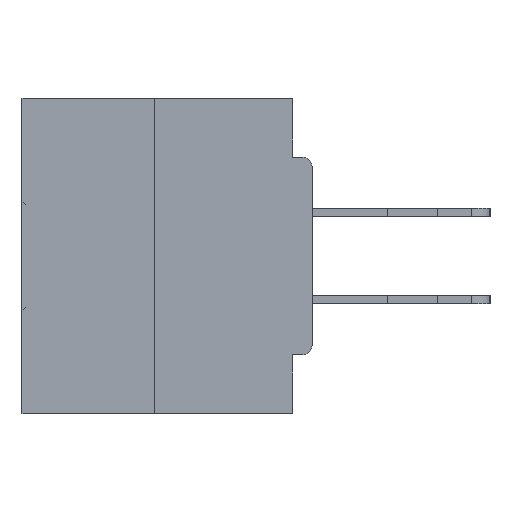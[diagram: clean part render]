
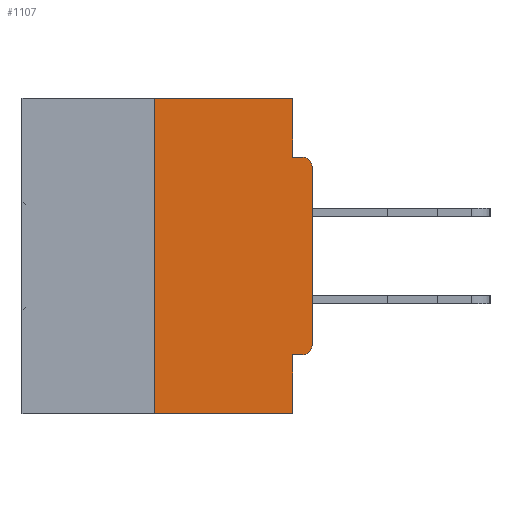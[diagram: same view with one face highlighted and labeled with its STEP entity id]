
A CAD part, left-side view. The second image highlights one B-rep face of the part: STEP entity #1107.
In plain terms, the highlighted planar face has unit normal (-1, 0, 0).
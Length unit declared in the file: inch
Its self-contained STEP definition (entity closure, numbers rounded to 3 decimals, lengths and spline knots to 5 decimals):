
#235 = VECTOR ( 'NONE', #36347, 39.37008 ) ;
#356 = VECTOR ( 'NONE', #8314, 39.37008 ) ;
#1107 = ADVANCED_FACE ( 'NONE', ( #28666 ), #30904, .F. ) ;
#2574 = CARTESIAN_POINT ( 'NONE',  ( 0., 0., -0.1085 ) ) ;
#3475 = DIRECTION ( 'NONE',  ( -1., 0., 0. ) ) ;
#3904 = VERTEX_POINT ( 'NONE', #31282 ) ;
#3958 = CARTESIAN_POINT ( 'NONE',  ( 0., 0.25, 0. ) ) ;
#4335 = DIRECTION ( 'NONE',  ( 1., 0., 0. ) ) ;
#4361 = ORIENTED_EDGE ( 'NONE', *, *, #42963, .T. ) ;
#5199 = AXIS2_PLACEMENT_3D ( 'NONE', #13605, #17382, #41067 ) ;
#5365 = VECTOR ( 'NONE', #28498, 39.37008 ) ;
#5649 = EDGE_CURVE ( 'NONE', #43180, #18150, #7087, .T. ) ;
#6334 = LINE ( 'NONE', #19129, #27477 ) ;
#7087 = LINE ( 'NONE', #37291, #10281 ) ;
#8314 = DIRECTION ( 'NONE',  ( 0., 1., 0. ) ) ;
#8985 = EDGE_CURVE ( 'NONE', #18150, #36351, #30164, .T. ) ;
#9647 = CARTESIAN_POINT ( 'NONE',  ( 0., 0.015, -0.4065 ) ) ;
#9792 = CARTESIAN_POINT ( 'NONE',  ( 0., 0.25, -0.5 ) ) ;
#9830 = EDGE_CURVE ( 'NONE', #14488, #33222, #6334, .T. ) ;
#10281 = VECTOR ( 'NONE', #16440, 39.37008 ) ;
#11903 = CIRCLE ( 'NONE', #30479, 0.015 ) ;
#11998 = LINE ( 'NONE', #24845, #24604 ) ;
#12230 = VERTEX_POINT ( 'NONE', #35843 ) ;
#13387 = EDGE_CURVE ( 'NONE', #33222, #12230, #39884, .T. ) ;
#13605 = CARTESIAN_POINT ( 'NONE',  ( 0., 0.015, -0.1085 ) ) ;
#13852 = DIRECTION ( 'NONE',  ( 0., 0., -1. ) ) ;
#14488 = VERTEX_POINT ( 'NONE', #9792 ) ;
#14993 = CARTESIAN_POINT ( 'NONE',  ( 0., 0.031, -0.5 ) ) ;
#14994 = EDGE_CURVE ( 'NONE', #16891, #36351, #37554, .T. ) ;
#15096 = CARTESIAN_POINT ( 'NONE',  ( 0., 0., -0.0935 ) ) ;
#16440 = DIRECTION ( 'NONE',  ( 0., 0., 1. ) ) ;
#16891 = VERTEX_POINT ( 'NONE', #23171 ) ;
#17126 = LINE ( 'NONE', #32949, #235 ) ;
#17382 = DIRECTION ( 'NONE',  ( -1., 0., 0. ) ) ;
#17494 = CARTESIAN_POINT ( 'NONE',  ( 0., 0.031, -0.5 ) ) ;
#18150 = VERTEX_POINT ( 'NONE', #2574 ) ;
#18290 = ORIENTED_EDGE ( 'NONE', *, *, #35519, .F. ) ;
#18487 = DIRECTION ( 'NONE',  ( 0., -1., 0. ) ) ;
#19129 = CARTESIAN_POINT ( 'NONE',  ( 0., 0.25, 0. ) ) ;
#20282 = ORIENTED_EDGE ( 'NONE', *, *, #8985, .T. ) ;
#23171 = CARTESIAN_POINT ( 'NONE',  ( 0., 0.031, -0.0935 ) ) ;
#24604 = VECTOR ( 'NONE', #39071, 39.37008 ) ;
#24845 = CARTESIAN_POINT ( 'NONE',  ( 0., 0.46, -0.5 ) ) ;
#25630 = EDGE_LOOP ( 'NONE', ( #43485, #36780, #4361, #28455, #18290, #30085, #40351, #20282, #36782, #35275 ) ) ;
#25725 = AXIS2_PLACEMENT_3D ( 'NONE', #31363, #4335, #37553 ) ;
#25814 = DIRECTION ( 'NONE',  ( 0., 0., 1. ) ) ;
#27001 = EDGE_CURVE ( 'NONE', #42233, #43180, #11903, .T. ) ;
#27413 = CARTESIAN_POINT ( 'NONE',  ( 0., 0.015, -0.3915 ) ) ;
#27477 = VECTOR ( 'NONE', #25814, 39.37008 ) ;
#28059 = VECTOR ( 'NONE', #31601, 39.37008 ) ;
#28455 = ORIENTED_EDGE ( 'NONE', *, *, #38924, .F. ) ;
#28498 = DIRECTION ( 'NONE',  ( 0., 0., -1. ) ) ;
#28666 = FACE_OUTER_BOUND ( 'NONE', #25630, .T. ) ;
#30085 = ORIENTED_EDGE ( 'NONE', *, *, #27001, .T. ) ;
#30164 = CIRCLE ( 'NONE', #5199, 0.015 ) ;
#30479 = AXIS2_PLACEMENT_3D ( 'NONE', #27413, #3475, #13852 ) ;
#30904 = PLANE ( 'NONE',  #25725 ) ;
#31282 = CARTESIAN_POINT ( 'NONE',  ( 0., 0.031, -0.4065 ) ) ;
#31363 = CARTESIAN_POINT ( 'NONE',  ( 0., 0.46, 0. ) ) ;
#31601 = DIRECTION ( 'NONE',  ( 0., -1., 0. ) ) ;
#32949 = CARTESIAN_POINT ( 'NONE',  ( 0., 0.031, 0. ) ) ;
#33222 = VERTEX_POINT ( 'NONE', #3958 ) ;
#33927 = CARTESIAN_POINT ( 'NONE',  ( 0., 0., -0.3915 ) ) ;
#35275 = ORIENTED_EDGE ( 'NONE', *, *, #36697, .F. ) ;
#35506 = LINE ( 'NONE', #17494, #5365 ) ;
#35519 = EDGE_CURVE ( 'NONE', #42233, #3904, #41652, .T. ) ;
#35843 = CARTESIAN_POINT ( 'NONE',  ( 0., 0.031, 0. ) ) ;
#36347 = DIRECTION ( 'NONE',  ( 0., 0., -1. ) ) ;
#36351 = VERTEX_POINT ( 'NONE', #39739 ) ;
#36697 = EDGE_CURVE ( 'NONE', #12230, #16891, #17126, .T. ) ;
#36780 = ORIENTED_EDGE ( 'NONE', *, *, #9830, .F. ) ;
#36782 = ORIENTED_EDGE ( 'NONE', *, *, #14994, .F. ) ;
#37291 = CARTESIAN_POINT ( 'NONE',  ( 0., 0., 0. ) ) ;
#37553 = DIRECTION ( 'NONE',  ( 0., 0., -1. ) ) ;
#37554 = LINE ( 'NONE', #15096, #28059 ) ;
#38172 = CARTESIAN_POINT ( 'NONE',  ( 0., 0., -0.4065 ) ) ;
#38635 = CARTESIAN_POINT ( 'NONE',  ( 0., 0.46, 0. ) ) ;
#38924 = EDGE_CURVE ( 'NONE', #3904, #42444, #35506, .T. ) ;
#39071 = DIRECTION ( 'NONE',  ( 0., -1., 0. ) ) ;
#39739 = CARTESIAN_POINT ( 'NONE',  ( 0., 0.015, -0.0935 ) ) ;
#39884 = LINE ( 'NONE', #38635, #42025 ) ;
#40351 = ORIENTED_EDGE ( 'NONE', *, *, #5649, .T. ) ;
#41067 = DIRECTION ( 'NONE',  ( 0., 0., -1. ) ) ;
#41652 = LINE ( 'NONE', #38172, #356 ) ;
#42025 = VECTOR ( 'NONE', #18487, 39.37008 ) ;
#42233 = VERTEX_POINT ( 'NONE', #9647 ) ;
#42444 = VERTEX_POINT ( 'NONE', #14993 ) ;
#42963 = EDGE_CURVE ( 'NONE', #14488, #42444, #11998, .T. ) ;
#43180 = VERTEX_POINT ( 'NONE', #33927 ) ;
#43485 = ORIENTED_EDGE ( 'NONE', *, *, #13387, .F. ) ;
